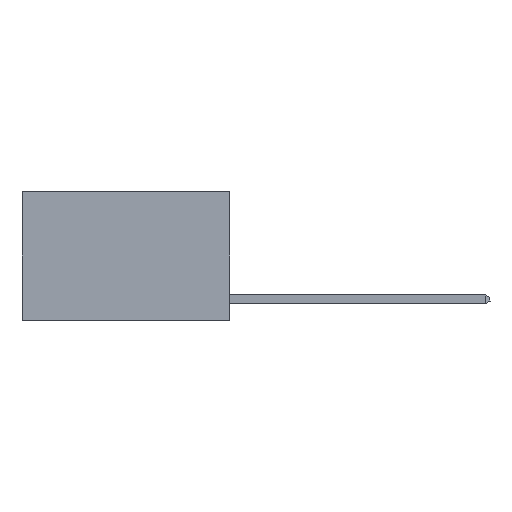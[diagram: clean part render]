
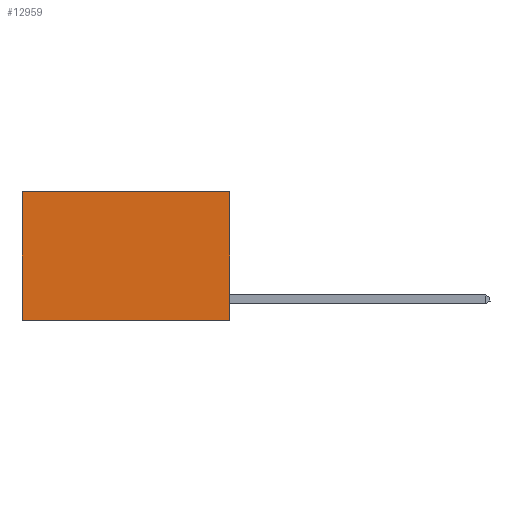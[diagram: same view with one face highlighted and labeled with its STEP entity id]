
A CAD part, left-side view. The second image highlights one B-rep face of the part: STEP entity #12959.
In plain terms, the highlighted planar face has unit normal (-1, 0, 0).
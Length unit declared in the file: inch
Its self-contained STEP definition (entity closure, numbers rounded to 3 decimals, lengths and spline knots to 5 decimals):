
#130 = VERTEX_POINT ( 'NONE', #4978 ) ;
#657 = VERTEX_POINT ( 'NONE', #18302 ) ;
#1427 = VERTEX_POINT ( 'NONE', #12049 ) ;
#2736 = VECTOR ( 'NONE', #9950, 39.37008 ) ;
#3455 = PLANE ( 'NONE',  #4419 ) ;
#3526 = LINE ( 'NONE', #24934, #14440 ) ;
#4419 = AXIS2_PLACEMENT_3D ( 'NONE', #9963, #18725, #5694 ) ;
#4978 = CARTESIAN_POINT ( 'NONE',  ( 0.2625, 0.6, -0.37 ) ) ;
#4986 = CARTESIAN_POINT ( 'NONE',  ( 0.2625, 0., 0. ) ) ;
#5076 = DIRECTION ( 'NONE',  ( 0., 1., 0. ) ) ;
#5545 = VECTOR ( 'NONE', #18933, 39.37008 ) ;
#5694 = DIRECTION ( 'NONE',  ( 0., 0., -1. ) ) ;
#7447 = ORIENTED_EDGE ( 'NONE', *, *, #16950, .F. ) ;
#8151 = VECTOR ( 'NONE', #5076, 39.37008 ) ;
#8218 = EDGE_CURVE ( 'NONE', #21479, #657, #3526, .T. ) ;
#8849 = CARTESIAN_POINT ( 'NONE',  ( 0.2625, 0., 0. ) ) ;
#9485 = LINE ( 'NONE', #4986, #8151 ) ;
#9950 = DIRECTION ( 'NONE',  ( 0., 1., 0. ) ) ;
#9963 = CARTESIAN_POINT ( 'NONE',  ( 0.2625, 0., 0. ) ) ;
#11449 = EDGE_CURVE ( 'NONE', #21479, #1427, #9485, .T. ) ;
#11836 = ORIENTED_EDGE ( 'NONE', *, *, #16404, .T. ) ;
#12049 = CARTESIAN_POINT ( 'NONE',  ( 0.2625, 0.6, 0. ) ) ;
#12959 = ADVANCED_FACE ( 'NONE', ( #13845 ), #3455, .F. ) ;
#13845 = FACE_OUTER_BOUND ( 'NONE', #26187, .T. ) ;
#14440 = VECTOR ( 'NONE', #27115, 39.37008 ) ;
#16404 = EDGE_CURVE ( 'NONE', #1427, #130, #22912, .T. ) ;
#16950 = EDGE_CURVE ( 'NONE', #657, #130, #20153, .T. ) ;
#18302 = CARTESIAN_POINT ( 'NONE',  ( 0.2625, 0., -0.37 ) ) ;
#18725 = DIRECTION ( 'NONE',  ( 1., 0., 0. ) ) ;
#18933 = DIRECTION ( 'NONE',  ( 0., 0., -1. ) ) ;
#19003 = ORIENTED_EDGE ( 'NONE', *, *, #8218, .F. ) ;
#20153 = LINE ( 'NONE', #20815, #2736 ) ;
#20815 = CARTESIAN_POINT ( 'NONE',  ( 0.2625, 0., -0.37 ) ) ;
#21479 = VERTEX_POINT ( 'NONE', #8849 ) ;
#22912 = LINE ( 'NONE', #23304, #5545 ) ;
#23304 = CARTESIAN_POINT ( 'NONE',  ( 0.2625, 0.6, 0. ) ) ;
#24934 = CARTESIAN_POINT ( 'NONE',  ( 0.2625, 0., 0. ) ) ;
#26108 = ORIENTED_EDGE ( 'NONE', *, *, #11449, .T. ) ;
#26187 = EDGE_LOOP ( 'NONE', ( #11836, #7447, #19003, #26108 ) ) ;
#27115 = DIRECTION ( 'NONE',  ( 0., 0., -1. ) ) ;
